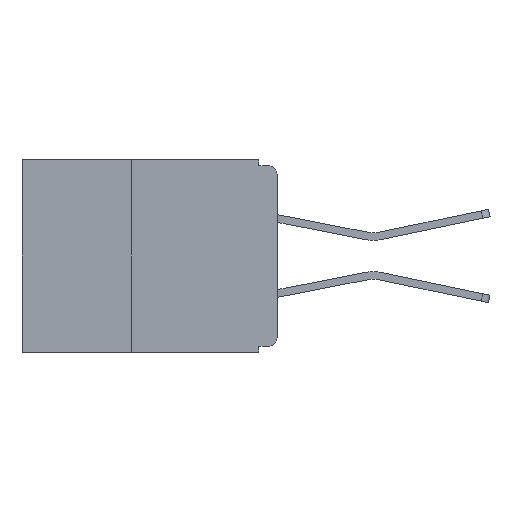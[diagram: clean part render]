
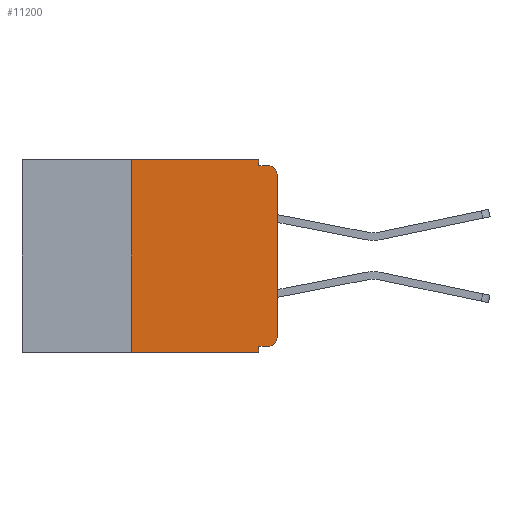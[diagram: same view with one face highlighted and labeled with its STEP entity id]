
A CAD part, left-side view. The second image highlights one B-rep face of the part: STEP entity #11200.
In plain terms, the highlighted planar face has unit normal (-1, 0, 0).
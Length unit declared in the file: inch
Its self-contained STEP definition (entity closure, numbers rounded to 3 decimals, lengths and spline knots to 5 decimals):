
#160 = EDGE_CURVE ( 'NONE', #20856, #15232, #22433, .T. ) ;
#529 = LINE ( 'NONE', #8875, #13602 ) ;
#912 = CARTESIAN_POINT ( 'NONE',  ( 0., 0., -0.32 ) ) ;
#1108 = DIRECTION ( 'NONE',  ( 0., 0., -1. ) ) ;
#1878 = VECTOR ( 'NONE', #27067, 39.37008 ) ;
#2252 = CARTESIAN_POINT ( 'NONE',  ( 0., 0.25, 0. ) ) ;
#2836 = DIRECTION ( 'NONE',  ( 0., -1., 0. ) ) ;
#2838 = VECTOR ( 'NONE', #2836, 39.37008 ) ;
#2919 = VECTOR ( 'NONE', #14062, 39.37008 ) ;
#2951 = EDGE_LOOP ( 'NONE', ( #9049, #3730, #17483, #13131, #31319, #5804, #26263, #13556, #27833, #15534 ) ) ;
#3344 = EDGE_CURVE ( 'NONE', #18269, #20856, #15907, .T. ) ;
#3553 = DIRECTION ( 'NONE',  ( 0., 1., 0. ) ) ;
#3730 = ORIENTED_EDGE ( 'NONE', *, *, #11590, .T. ) ;
#3756 = EDGE_CURVE ( 'NONE', #26257, #7847, #16670, .T. ) ;
#4062 = EDGE_CURVE ( 'NONE', #5581, #26257, #13883, .T. ) ;
#5581 = VERTEX_POINT ( 'NONE', #13239 ) ;
#5804 = ORIENTED_EDGE ( 'NONE', *, *, #29158, .F. ) ;
#5875 = VERTEX_POINT ( 'NONE', #6854 ) ;
#5920 = VERTEX_POINT ( 'NONE', #6152 ) ;
#6152 = CARTESIAN_POINT ( 'NONE',  ( 0., 0.031, -0.32 ) ) ;
#6844 = LINE ( 'NONE', #19894, #19721 ) ;
#6854 = CARTESIAN_POINT ( 'NONE',  ( 0., 0.25, -0.33 ) ) ;
#7336 = EDGE_CURVE ( 'NONE', #10566, #18269, #6844, .T. ) ;
#7847 = VERTEX_POINT ( 'NONE', #19433 ) ;
#7947 = CARTESIAN_POINT ( 'NONE',  ( 0., 0.437, -0.33 ) ) ;
#8205 = CIRCLE ( 'NONE', #24039, 0.015 ) ;
#8875 = CARTESIAN_POINT ( 'NONE',  ( 0., 0.031, -0.33 ) ) ;
#9049 = ORIENTED_EDGE ( 'NONE', *, *, #3756, .T. ) ;
#9161 = CARTESIAN_POINT ( 'NONE',  ( 0., 0.015, -0.025 ) ) ;
#9753 = LINE ( 'NONE', #7947, #2838 ) ;
#9935 = CARTESIAN_POINT ( 'NONE',  ( 0., 0., 0. ) ) ;
#10322 = EDGE_CURVE ( 'NONE', #5920, #13969, #529, .T. ) ;
#10566 = VERTEX_POINT ( 'NONE', #2252 ) ;
#11200 = ADVANCED_FACE ( 'NONE', ( #19480 ), #12464, .F. ) ;
#11590 = EDGE_CURVE ( 'NONE', #7847, #15232, #8205, .T. ) ;
#11763 = DIRECTION ( 'NONE',  ( 0., 0., -1. ) ) ;
#12464 = PLANE ( 'NONE',  #26369 ) ;
#12877 = VECTOR ( 'NONE', #32890, 39.37008 ) ;
#13131 = ORIENTED_EDGE ( 'NONE', *, *, #3344, .F. ) ;
#13239 = CARTESIAN_POINT ( 'NONE',  ( 0., 0.015, -0.32 ) ) ;
#13556 = ORIENTED_EDGE ( 'NONE', *, *, #10322, .F. ) ;
#13602 = VECTOR ( 'NONE', #1108, 39.37008 ) ;
#13610 = CARTESIAN_POINT ( 'NONE',  ( 0., 0.015, -0.01 ) ) ;
#13883 = CIRCLE ( 'NONE', #29136, 0.015 ) ;
#13969 = VERTEX_POINT ( 'NONE', #23334 ) ;
#14062 = DIRECTION ( 'NONE',  ( 0., 0., 1. ) ) ;
#15040 = DIRECTION ( 'NONE',  ( 1., 0., 0. ) ) ;
#15232 = VERTEX_POINT ( 'NONE', #13610 ) ;
#15534 = ORIENTED_EDGE ( 'NONE', *, *, #4062, .T. ) ;
#15907 = LINE ( 'NONE', #18650, #22658 ) ;
#16670 = LINE ( 'NONE', #9935, #2919 ) ;
#17466 = DIRECTION ( 'NONE',  ( 0., 0., -1. ) ) ;
#17483 = ORIENTED_EDGE ( 'NONE', *, *, #160, .F. ) ;
#18269 = VERTEX_POINT ( 'NONE', #28030 ) ;
#18650 = CARTESIAN_POINT ( 'NONE',  ( 0., 0.031, 0. ) ) ;
#19014 = CARTESIAN_POINT ( 'NONE',  ( 0., 0., -0.01 ) ) ;
#19038 = EDGE_CURVE ( 'NONE', #5875, #13969, #9753, .T. ) ;
#19433 = CARTESIAN_POINT ( 'NONE',  ( 0., 0., -0.025 ) ) ;
#19480 = FACE_OUTER_BOUND ( 'NONE', #2951, .T. ) ;
#19721 = VECTOR ( 'NONE', #25012, 39.37008 ) ;
#19894 = CARTESIAN_POINT ( 'NONE',  ( 0., 0.437, 0. ) ) ;
#20856 = VERTEX_POINT ( 'NONE', #28390 ) ;
#21720 = CARTESIAN_POINT ( 'NONE',  ( 0., 0., -0.305 ) ) ;
#22385 = EDGE_CURVE ( 'NONE', #5581, #5920, #29082, .T. ) ;
#22433 = LINE ( 'NONE', #19014, #1878 ) ;
#22658 = VECTOR ( 'NONE', #17466, 39.37008 ) ;
#22875 = CARTESIAN_POINT ( 'NONE',  ( 0., 0.25, -0.33 ) ) ;
#23334 = CARTESIAN_POINT ( 'NONE',  ( 0., 0.031, -0.33 ) ) ;
#24039 = AXIS2_PLACEMENT_3D ( 'NONE', #9161, #27007, #11763 ) ;
#25012 = DIRECTION ( 'NONE',  ( 0., -1., 0. ) ) ;
#26257 = VERTEX_POINT ( 'NONE', #21720 ) ;
#26263 = ORIENTED_EDGE ( 'NONE', *, *, #19038, .T. ) ;
#26369 = AXIS2_PLACEMENT_3D ( 'NONE', #27683, #15040, #32621 ) ;
#27007 = DIRECTION ( 'NONE',  ( -1., 0., 0. ) ) ;
#27067 = DIRECTION ( 'NONE',  ( 0., -1., 0. ) ) ;
#27683 = CARTESIAN_POINT ( 'NONE',  ( 0., 0.437, 0. ) ) ;
#27833 = ORIENTED_EDGE ( 'NONE', *, *, #22385, .F. ) ;
#28030 = CARTESIAN_POINT ( 'NONE',  ( 0., 0.031, 0. ) ) ;
#28390 = CARTESIAN_POINT ( 'NONE',  ( 0., 0.031, -0.01 ) ) ;
#29082 = LINE ( 'NONE', #912, #29855 ) ;
#29136 = AXIS2_PLACEMENT_3D ( 'NONE', #31899, #31888, #31861 ) ;
#29158 = EDGE_CURVE ( 'NONE', #5875, #10566, #32936, .T. ) ;
#29855 = VECTOR ( 'NONE', #3553, 39.37008 ) ;
#31319 = ORIENTED_EDGE ( 'NONE', *, *, #7336, .F. ) ;
#31861 = DIRECTION ( 'NONE',  ( 0., 0., -1. ) ) ;
#31888 = DIRECTION ( 'NONE',  ( -1., 0., 0. ) ) ;
#31899 = CARTESIAN_POINT ( 'NONE',  ( 0., 0.015, -0.305 ) ) ;
#32621 = DIRECTION ( 'NONE',  ( 0., 0., -1. ) ) ;
#32890 = DIRECTION ( 'NONE',  ( 0., 0., 1. ) ) ;
#32936 = LINE ( 'NONE', #22875, #12877 ) ;
